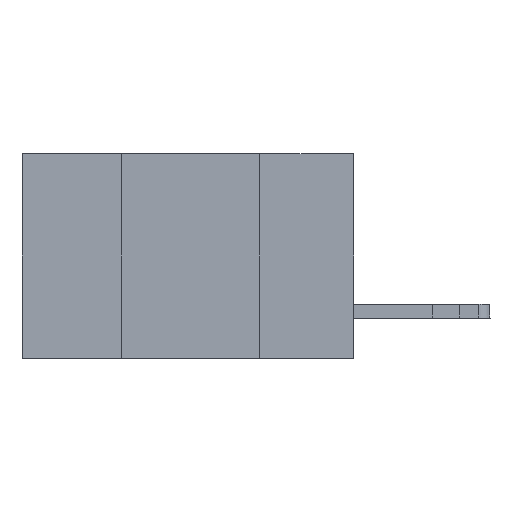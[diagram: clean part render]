
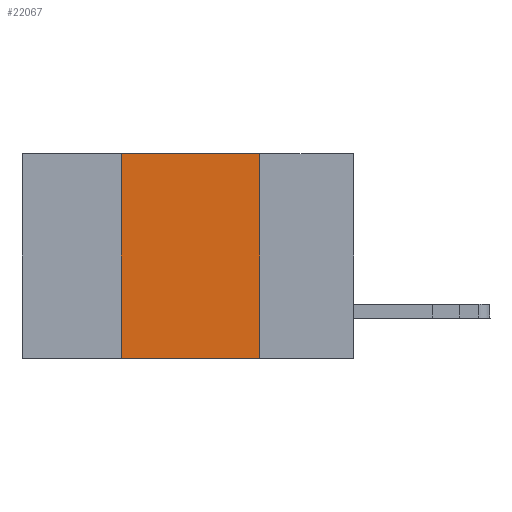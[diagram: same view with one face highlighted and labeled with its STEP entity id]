
A CAD part, left-side view. The second image highlights one B-rep face of the part: STEP entity #22067.
In plain terms, the highlighted planar face has unit normal (-1, 0, 0).
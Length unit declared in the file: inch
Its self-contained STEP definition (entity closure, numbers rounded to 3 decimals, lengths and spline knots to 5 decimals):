
#20 = VECTOR ( 'NONE', #8589, 39.37008 ) ;
#512 = DIRECTION ( 'NONE',  ( 0., -1., 0. ) ) ;
#760 = LINE ( 'NONE', #10797, #20 ) ;
#924 = DIRECTION ( 'NONE',  ( 0., 0., -1. ) ) ;
#2266 = VECTOR ( 'NONE', #27408, 39.37008 ) ;
#2736 = CARTESIAN_POINT ( 'NONE',  ( 0., 0.17, 0. ) ) ;
#4858 = CARTESIAN_POINT ( 'NONE',  ( 0., 0.42, 0. ) ) ;
#5128 = LINE ( 'NONE', #17150, #22699 ) ;
#7776 = LINE ( 'NONE', #13814, #2266 ) ;
#8541 = CARTESIAN_POINT ( 'NONE',  ( 0., 0.42, -0.37 ) ) ;
#8589 = DIRECTION ( 'NONE',  ( 0., 0., 1. ) ) ;
#9830 = LINE ( 'NONE', #28079, #15230 ) ;
#10089 = VERTEX_POINT ( 'NONE', #2736 ) ;
#10797 = CARTESIAN_POINT ( 'NONE',  ( 0., 0.42, 0. ) ) ;
#12231 = DIRECTION ( 'NONE',  ( 1., 0., 0. ) ) ;
#13814 = CARTESIAN_POINT ( 'NONE',  ( 0., 0.6, -0.37 ) ) ;
#13861 = EDGE_CURVE ( 'NONE', #16922, #18148, #7776, .T. ) ;
#14841 = FACE_OUTER_BOUND ( 'NONE', #24770, .T. ) ;
#14934 = ORIENTED_EDGE ( 'NONE', *, *, #15361, .F. ) ;
#15230 = VECTOR ( 'NONE', #512, 39.37008 ) ;
#15361 = EDGE_CURVE ( 'NONE', #10089, #18148, #5128, .T. ) ;
#16512 = CARTESIAN_POINT ( 'NONE',  ( 0., 0.17, -0.37 ) ) ;
#16922 = VERTEX_POINT ( 'NONE', #8541 ) ;
#17150 = CARTESIAN_POINT ( 'NONE',  ( 0., 0.17, 0. ) ) ;
#18148 = VERTEX_POINT ( 'NONE', #16512 ) ;
#19761 = EDGE_CURVE ( 'NONE', #16922, #26202, #760, .T. ) ;
#20177 = ORIENTED_EDGE ( 'NONE', *, *, #21411, .F. ) ;
#21260 = ORIENTED_EDGE ( 'NONE', *, *, #19761, .F. ) ;
#21292 = PLANE ( 'NONE',  #27231 ) ;
#21411 = EDGE_CURVE ( 'NONE', #26202, #10089, #9830, .T. ) ;
#22067 = ADVANCED_FACE ( 'NONE', ( #14841 ), #21292, .F. ) ;
#22699 = VECTOR ( 'NONE', #924, 39.37008 ) ;
#24770 = EDGE_LOOP ( 'NONE', ( #14934, #20177, #21260, #29144 ) ) ;
#25857 = CARTESIAN_POINT ( 'NONE',  ( 0., 0.6, 0. ) ) ;
#26202 = VERTEX_POINT ( 'NONE', #4858 ) ;
#27231 = AXIS2_PLACEMENT_3D ( 'NONE', #25857, #12231, #28145 ) ;
#27408 = DIRECTION ( 'NONE',  ( 0., -1., 0. ) ) ;
#28079 = CARTESIAN_POINT ( 'NONE',  ( 0., 0.6, 0. ) ) ;
#28145 = DIRECTION ( 'NONE',  ( 0., 0., -1. ) ) ;
#29144 = ORIENTED_EDGE ( 'NONE', *, *, #13861, .T. ) ;
